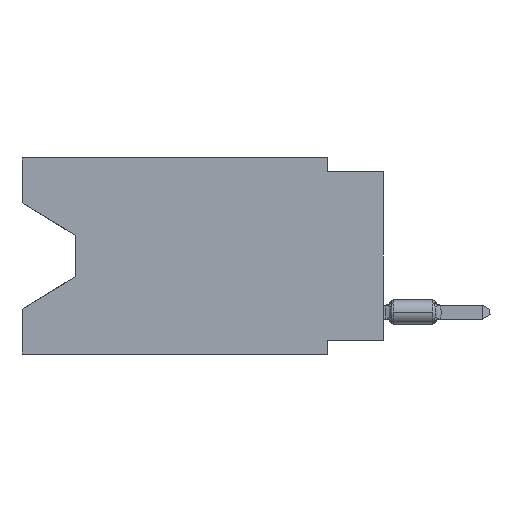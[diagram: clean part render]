
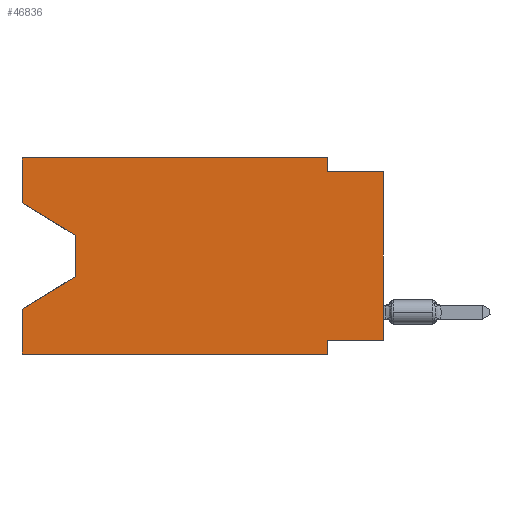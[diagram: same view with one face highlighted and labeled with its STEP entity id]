
A CAD part, left-side view. The second image highlights one B-rep face of the part: STEP entity #46836.
In plain terms, the highlighted planar face has unit normal (-1, 0, 0).
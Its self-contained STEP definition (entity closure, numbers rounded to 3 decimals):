
#1170 = CARTESIAN_POINT ( 'NONE',  ( 0., 13.97, -5.385 ) ) ;
#1564 = LINE ( 'NONE', #29515, #55209 ) ;
#1924 = AXIS2_PLACEMENT_3D ( 'NONE', #57111, #62655, #8559 ) ;
#2429 = DIRECTION ( 'NONE',  ( 0., 0., -1. ) ) ;
#2830 = VERTEX_POINT ( 'NONE', #87922 ) ;
#4638 = EDGE_CURVE ( 'NONE', #4690, #68932, #52458, .T. ) ;
#4690 = VERTEX_POINT ( 'NONE', #73075 ) ;
#6777 = PLANE ( 'NONE',  #1924 ) ;
#7773 = LINE ( 'NONE', #76951, #87619 ) ;
#8559 = DIRECTION ( 'NONE',  ( 0., 0., -1. ) ) ;
#9807 = CARTESIAN_POINT ( 'NONE',  ( 0., 2.54, 0. ) ) ;
#13578 = VERTEX_POINT ( 'NONE', #14307 ) ;
#14190 = CARTESIAN_POINT ( 'NONE',  ( 0., 0., -8.255 ) ) ;
#14307 = CARTESIAN_POINT ( 'NONE',  ( 0., 16.383, -2.038 ) ) ;
#16927 = VECTOR ( 'NONE', #28242, 1000. ) ;
#16985 = ORIENTED_EDGE ( 'NONE', *, *, #60168, .F. ) ;
#19046 = VECTOR ( 'NONE', #62774, 1000. ) ;
#19762 = EDGE_CURVE ( 'NONE', #24058, #39159, #86072, .T. ) ;
#20182 = LINE ( 'NONE', #69213, #19046 ) ;
#21523 = DIRECTION ( 'NONE',  ( 0., -1., 0. ) ) ;
#22537 = VECTOR ( 'NONE', #2429, 1000. ) ;
#22572 = ORIENTED_EDGE ( 'NONE', *, *, #84996, .F. ) ;
#23315 = CARTESIAN_POINT ( 'NONE',  ( 0., 2.54, 0. ) ) ;
#23611 = DIRECTION ( 'NONE',  ( 0., 0., 1. ) ) ;
#23751 = VECTOR ( 'NONE', #62772, 1000. ) ;
#24058 = VERTEX_POINT ( 'NONE', #9807 ) ;
#26386 = VERTEX_POINT ( 'NONE', #86273 ) ;
#28242 = DIRECTION ( 'NONE',  ( 0., -1., 0. ) ) ;
#29515 = CARTESIAN_POINT ( 'NONE',  ( 0., 2.54, -8.89 ) ) ;
#29928 = VECTOR ( 'NONE', #33830, 1000. ) ;
#29984 = EDGE_CURVE ( 'NONE', #2830, #40177, #51437, .T. ) ;
#30678 = EDGE_CURVE ( 'NONE', #13578, #2830, #61310, .T. ) ;
#31045 = ORIENTED_EDGE ( 'NONE', *, *, #30678, .T. ) ;
#32979 = EDGE_CURVE ( 'NONE', #40177, #68932, #82861, .T. ) ;
#33830 = DIRECTION ( 'NONE',  ( 0., -0.855, -0.519 ) ) ;
#36635 = DIRECTION ( 'NONE',  ( 0., 0., -1. ) ) ;
#37367 = EDGE_LOOP ( 'NONE', ( #31045, #81216, #48434, #83083, #41866, #38125, #22572, #88507, #16985, #71011, #57548, #44965 ) ) ;
#38125 = ORIENTED_EDGE ( 'NONE', *, *, #63789, .F. ) ;
#39159 = VERTEX_POINT ( 'NONE', #54208 ) ;
#39813 = CARTESIAN_POINT ( 'NONE',  ( 0., 16.383, 0. ) ) ;
#40070 = CARTESIAN_POINT ( 'NONE',  ( 0., 16.383, -6.852 ) ) ;
#40177 = VERTEX_POINT ( 'NONE', #1170 ) ;
#41707 = CARTESIAN_POINT ( 'NONE',  ( 0., 0., -0.635 ) ) ;
#41866 = ORIENTED_EDGE ( 'NONE', *, *, #89612, .T. ) ;
#44965 = ORIENTED_EDGE ( 'NONE', *, *, #49421, .F. ) ;
#46687 = DIRECTION ( 'NONE',  ( 0., 0.855, -0.519 ) ) ;
#46836 = ADVANCED_FACE ( 'NONE', ( #49379 ), #6777, .F. ) ;
#47088 = VECTOR ( 'NONE', #72594, 1000. ) ;
#47282 = CARTESIAN_POINT ( 'NONE',  ( 0., 16.383, 0. ) ) ;
#48434 = ORIENTED_EDGE ( 'NONE', *, *, #32979, .T. ) ;
#49379 = FACE_OUTER_BOUND ( 'NONE', #37367, .T. ) ;
#49421 = EDGE_CURVE ( 'NONE', #13578, #65520, #55242, .T. ) ;
#51109 = CARTESIAN_POINT ( 'NONE',  ( 0., 2.54, -8.255 ) ) ;
#51437 = LINE ( 'NONE', #63847, #22537 ) ;
#52458 = LINE ( 'NONE', #86813, #54183 ) ;
#53650 = VECTOR ( 'NONE', #46687, 1000. ) ;
#54183 = VECTOR ( 'NONE', #23611, 1000. ) ;
#54208 = CARTESIAN_POINT ( 'NONE',  ( 0., 2.54, -0.635 ) ) ;
#54914 = CARTESIAN_POINT ( 'NONE',  ( 0., 13.97, -5.385 ) ) ;
#55209 = VECTOR ( 'NONE', #57446, 1000. ) ;
#55242 = LINE ( 'NONE', #39813, #84073 ) ;
#57111 = CARTESIAN_POINT ( 'NONE',  ( 0., 16.383, 0. ) ) ;
#57269 = EDGE_CURVE ( 'NONE', #67248, #72310, #20182, .T. ) ;
#57446 = DIRECTION ( 'NONE',  ( 0., 0., -1. ) ) ;
#57548 = ORIENTED_EDGE ( 'NONE', *, *, #81678, .F. ) ;
#59157 = VECTOR ( 'NONE', #36635, 1000. ) ;
#60168 = EDGE_CURVE ( 'NONE', #39159, #72310, #82935, .T. ) ;
#61310 = LINE ( 'NONE', #67274, #29928 ) ;
#62655 = DIRECTION ( 'NONE',  ( 1., 0., 0. ) ) ;
#62772 = DIRECTION ( 'NONE',  ( 0., -1., 0. ) ) ;
#62774 = DIRECTION ( 'NONE',  ( 0., 0., 1. ) ) ;
#63789 = EDGE_CURVE ( 'NONE', #80371, #26386, #1564, .T. ) ;
#63847 = CARTESIAN_POINT ( 'NONE',  ( 0., 13.97, -3.505 ) ) ;
#64865 = CARTESIAN_POINT ( 'NONE',  ( 0., 16.383, -8.89 ) ) ;
#65520 = VERTEX_POINT ( 'NONE', #47282 ) ;
#67248 = VERTEX_POINT ( 'NONE', #14190 ) ;
#67274 = CARTESIAN_POINT ( 'NONE',  ( 0., 16.383, -2.038 ) ) ;
#68932 = VERTEX_POINT ( 'NONE', #40070 ) ;
#69213 = CARTESIAN_POINT ( 'NONE',  ( 0., 0., 0. ) ) ;
#71011 = ORIENTED_EDGE ( 'NONE', *, *, #19762, .F. ) ;
#71309 = LINE ( 'NONE', #64865, #16927 ) ;
#72310 = VERTEX_POINT ( 'NONE', #77942 ) ;
#72594 = DIRECTION ( 'NONE',  ( 0., 1., 0. ) ) ;
#73075 = CARTESIAN_POINT ( 'NONE',  ( 0., 16.383, -8.89 ) ) ;
#73491 = LINE ( 'NONE', #88132, #47088 ) ;
#76951 = CARTESIAN_POINT ( 'NONE',  ( 0., 16.383, 0. ) ) ;
#77942 = CARTESIAN_POINT ( 'NONE',  ( 0., 0., -0.635 ) ) ;
#80371 = VERTEX_POINT ( 'NONE', #51109 ) ;
#81216 = ORIENTED_EDGE ( 'NONE', *, *, #29984, .T. ) ;
#81678 = EDGE_CURVE ( 'NONE', #65520, #24058, #7773, .T. ) ;
#82861 = LINE ( 'NONE', #54914, #53650 ) ;
#82935 = LINE ( 'NONE', #41707, #23751 ) ;
#83083 = ORIENTED_EDGE ( 'NONE', *, *, #4638, .F. ) ;
#84073 = VECTOR ( 'NONE', #88353, 1000. ) ;
#84996 = EDGE_CURVE ( 'NONE', #67248, #80371, #73491, .T. ) ;
#86072 = LINE ( 'NONE', #23315, #59157 ) ;
#86273 = CARTESIAN_POINT ( 'NONE',  ( 0., 2.54, -8.89 ) ) ;
#86813 = CARTESIAN_POINT ( 'NONE',  ( 0., 16.383, 0. ) ) ;
#87619 = VECTOR ( 'NONE', #21523, 1000. ) ;
#87922 = CARTESIAN_POINT ( 'NONE',  ( 0., 13.97, -3.505 ) ) ;
#88132 = CARTESIAN_POINT ( 'NONE',  ( 0., 0., -8.255 ) ) ;
#88353 = DIRECTION ( 'NONE',  ( 0., 0., 1. ) ) ;
#88507 = ORIENTED_EDGE ( 'NONE', *, *, #57269, .T. ) ;
#89612 = EDGE_CURVE ( 'NONE', #4690, #26386, #71309, .T. ) ;
